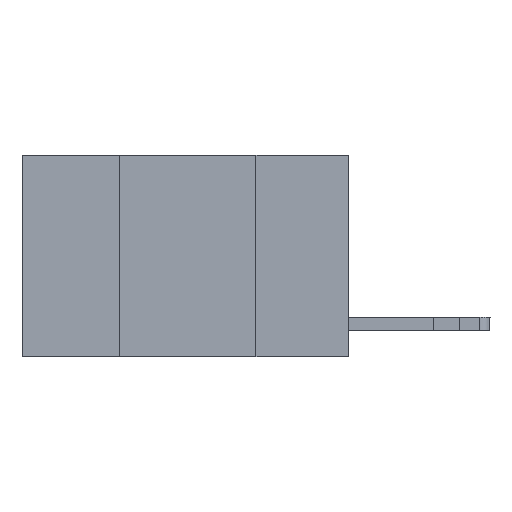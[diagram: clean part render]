
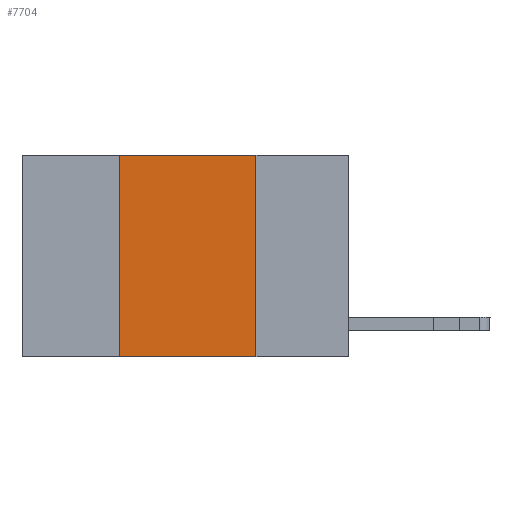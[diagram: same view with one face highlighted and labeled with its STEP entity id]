
A CAD part, left-side view. The second image highlights one B-rep face of the part: STEP entity #7704.
In plain terms, the highlighted planar face has unit normal (-1, 0, 0).
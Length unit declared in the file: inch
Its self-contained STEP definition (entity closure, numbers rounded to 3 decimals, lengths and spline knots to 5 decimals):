
#377 = DIRECTION ( 'NONE',  ( 0., -1., 0. ) ) ;
#1026 = EDGE_CURVE ( 'NONE', #7246, #15307, #9165, .T. ) ;
#1805 = CARTESIAN_POINT ( 'NONE',  ( 0., 0.17, -0.37 ) ) ;
#1816 = CARTESIAN_POINT ( 'NONE',  ( 0., 0.6, 0. ) ) ;
#2044 = VECTOR ( 'NONE', #10455, 39.37008 ) ;
#2454 = CARTESIAN_POINT ( 'NONE',  ( 0., 0.42, 0. ) ) ;
#3318 = LINE ( 'NONE', #5348, #14124 ) ;
#3905 = EDGE_CURVE ( 'NONE', #4951, #15307, #3318, .T. ) ;
#3921 = AXIS2_PLACEMENT_3D ( 'NONE', #1816, #15982, #7542 ) ;
#4340 = CARTESIAN_POINT ( 'NONE',  ( 0., 0.6, -0.37 ) ) ;
#4685 = CARTESIAN_POINT ( 'NONE',  ( 0., 0.6, 0. ) ) ;
#4951 = VERTEX_POINT ( 'NONE', #5079 ) ;
#5079 = CARTESIAN_POINT ( 'NONE',  ( 0., 0.17, 0. ) ) ;
#5348 = CARTESIAN_POINT ( 'NONE',  ( 0., 0.17, 0. ) ) ;
#5431 = DIRECTION ( 'NONE',  ( 0., 0., 1. ) ) ;
#7246 = VERTEX_POINT ( 'NONE', #12146 ) ;
#7542 = DIRECTION ( 'NONE',  ( 0., 0., -1. ) ) ;
#7683 = EDGE_CURVE ( 'NONE', #8559, #4951, #17409, .T. ) ;
#7704 = ADVANCED_FACE ( 'NONE', ( #9947 ), #14518, .F. ) ;
#8559 = VERTEX_POINT ( 'NONE', #2454 ) ;
#9128 = EDGE_LOOP ( 'NONE', ( #10398, #13490, #15045, #15266 ) ) ;
#9165 = LINE ( 'NONE', #4340, #2044 ) ;
#9947 = FACE_OUTER_BOUND ( 'NONE', #9128, .T. ) ;
#10398 = ORIENTED_EDGE ( 'NONE', *, *, #3905, .F. ) ;
#10455 = DIRECTION ( 'NONE',  ( 0., -1., 0. ) ) ;
#11556 = VECTOR ( 'NONE', #5431, 39.37008 ) ;
#12146 = CARTESIAN_POINT ( 'NONE',  ( 0., 0.42, -0.37 ) ) ;
#13490 = ORIENTED_EDGE ( 'NONE', *, *, #7683, .F. ) ;
#13680 = VECTOR ( 'NONE', #377, 39.37008 ) ;
#14124 = VECTOR ( 'NONE', #15186, 39.37008 ) ;
#14518 = PLANE ( 'NONE',  #3921 ) ;
#15045 = ORIENTED_EDGE ( 'NONE', *, *, #15827, .F. ) ;
#15186 = DIRECTION ( 'NONE',  ( 0., 0., -1. ) ) ;
#15266 = ORIENTED_EDGE ( 'NONE', *, *, #1026, .T. ) ;
#15307 = VERTEX_POINT ( 'NONE', #1805 ) ;
#15722 = LINE ( 'NONE', #18065, #11556 ) ;
#15827 = EDGE_CURVE ( 'NONE', #7246, #8559, #15722, .T. ) ;
#15982 = DIRECTION ( 'NONE',  ( 1., 0., 0. ) ) ;
#17409 = LINE ( 'NONE', #4685, #13680 ) ;
#18065 = CARTESIAN_POINT ( 'NONE',  ( 0., 0.42, 0. ) ) ;
